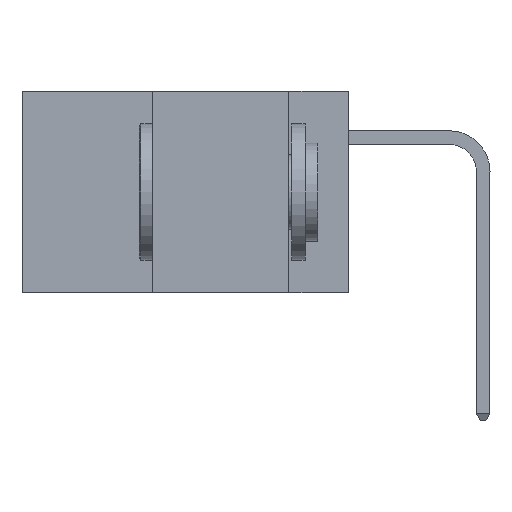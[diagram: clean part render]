
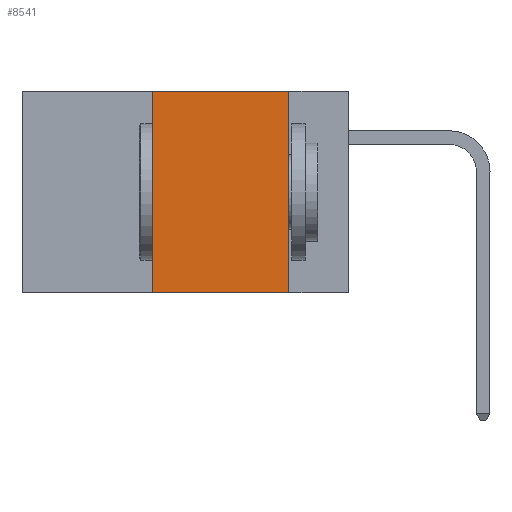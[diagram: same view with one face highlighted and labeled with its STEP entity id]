
A CAD part, left-side view. The second image highlights one B-rep face of the part: STEP entity #8541.
In plain terms, the highlighted planar face has unit normal (-1, 0, 0).
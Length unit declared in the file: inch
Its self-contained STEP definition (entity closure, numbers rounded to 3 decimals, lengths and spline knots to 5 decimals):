
#351 = CARTESIAN_POINT ( 'NONE',  ( 0., 0.6, 0. ) ) ;
#633 = CARTESIAN_POINT ( 'NONE',  ( 0., 0.36, 0. ) ) ;
#976 = ORIENTED_EDGE ( 'NONE', *, *, #7699, .T. ) ;
#1375 = VERTEX_POINT ( 'NONE', #7906 ) ;
#1601 = ORIENTED_EDGE ( 'NONE', *, *, #14104, .F. ) ;
#1606 = VECTOR ( 'NONE', #9491, 39.37008 ) ;
#1893 = ORIENTED_EDGE ( 'NONE', *, *, #9814, .F. ) ;
#2055 = CARTESIAN_POINT ( 'NONE',  ( 0., 0.11, -0.37 ) ) ;
#2426 = EDGE_CURVE ( 'NONE', #5817, #10429, #14753, .T. ) ;
#2819 = DIRECTION ( 'NONE',  ( 1., 0., 0. ) ) ;
#2937 = DIRECTION ( 'NONE',  ( 0., -1., 0. ) ) ;
#5369 = DIRECTION ( 'NONE',  ( 0., 0., -1. ) ) ;
#5400 = CARTESIAN_POINT ( 'NONE',  ( 0., 0.36, -0.37 ) ) ;
#5817 = VERTEX_POINT ( 'NONE', #5400 ) ;
#6681 = VECTOR ( 'NONE', #13827, 39.37008 ) ;
#6911 = CARTESIAN_POINT ( 'NONE',  ( 0., 0.6, -0.37 ) ) ;
#7364 = FACE_OUTER_BOUND ( 'NONE', #11431, .T. ) ;
#7699 = EDGE_CURVE ( 'NONE', #5817, #11846, #9744, .T. ) ;
#7906 = CARTESIAN_POINT ( 'NONE',  ( 0., 0.11, 0. ) ) ;
#8541 = ADVANCED_FACE ( 'NONE', ( #7364 ), #13247, .F. ) ;
#9491 = DIRECTION ( 'NONE',  ( 0., 0., 1. ) ) ;
#9644 = CARTESIAN_POINT ( 'NONE',  ( 0., 0.36, 0. ) ) ;
#9744 = LINE ( 'NONE', #6911, #6681 ) ;
#9814 = EDGE_CURVE ( 'NONE', #10429, #1375, #10404, .T. ) ;
#9917 = CARTESIAN_POINT ( 'NONE',  ( 0., 0.6, 0. ) ) ;
#10045 = ORIENTED_EDGE ( 'NONE', *, *, #2426, .F. ) ;
#10404 = LINE ( 'NONE', #9917, #13839 ) ;
#10429 = VERTEX_POINT ( 'NONE', #633 ) ;
#11011 = DIRECTION ( 'NONE',  ( 0., 0., -1. ) ) ;
#11431 = EDGE_LOOP ( 'NONE', ( #1601, #1893, #10045, #976 ) ) ;
#11611 = VECTOR ( 'NONE', #5369, 39.37008 ) ;
#11778 = AXIS2_PLACEMENT_3D ( 'NONE', #351, #2819, #11011 ) ;
#11846 = VERTEX_POINT ( 'NONE', #2055 ) ;
#13247 = PLANE ( 'NONE',  #11778 ) ;
#13463 = CARTESIAN_POINT ( 'NONE',  ( 0., 0.11, 0. ) ) ;
#13827 = DIRECTION ( 'NONE',  ( 0., -1., 0. ) ) ;
#13839 = VECTOR ( 'NONE', #2937, 39.37008 ) ;
#14104 = EDGE_CURVE ( 'NONE', #1375, #11846, #14261, .T. ) ;
#14261 = LINE ( 'NONE', #13463, #11611 ) ;
#14753 = LINE ( 'NONE', #9644, #1606 ) ;
